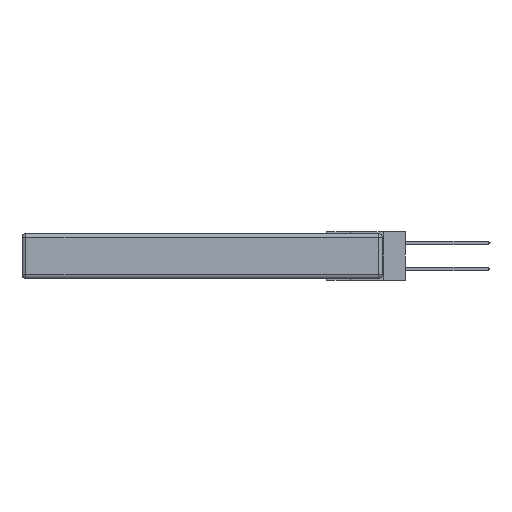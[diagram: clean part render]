
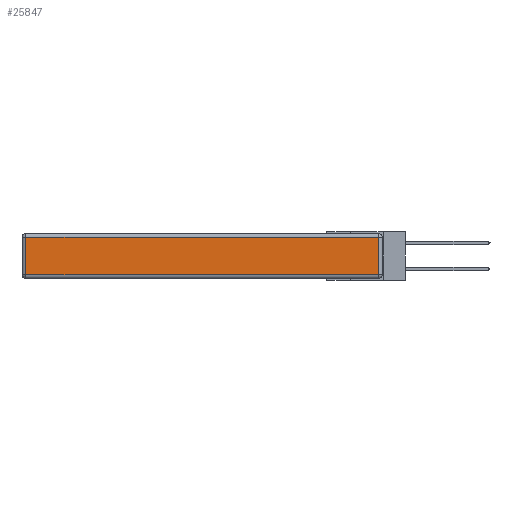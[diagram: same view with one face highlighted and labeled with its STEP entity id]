
A CAD part, left-side view. The second image highlights one B-rep face of the part: STEP entity #25847.
In plain terms, the highlighted planar face has unit normal (-1, 0, 0).
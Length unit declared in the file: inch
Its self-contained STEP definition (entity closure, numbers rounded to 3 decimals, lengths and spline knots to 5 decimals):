
#331 = DIRECTION ( 'NONE',  ( -1., 0., 0. ) ) ;
#1033 = CARTESIAN_POINT ( 'NONE',  ( 0., 0.03, -0.03 ) ) ;
#2004 = EDGE_CURVE ( 'NONE', #24551, #17968, #24460, .T. ) ;
#2163 = VERTEX_POINT ( 'NONE', #9667 ) ;
#3078 = FACE_OUTER_BOUND ( 'NONE', #28314, .T. ) ;
#4848 = VECTOR ( 'NONE', #13056, 39.37008 ) ;
#5954 = DIRECTION ( 'NONE',  ( 0., 0., 1. ) ) ;
#6379 = ORIENTED_EDGE ( 'NONE', *, *, #10879, .T. ) ;
#6501 = DIRECTION ( 'NONE',  ( 0., 1., 0. ) ) ;
#6529 = CARTESIAN_POINT ( 'NONE',  ( 0., 2.72, -0.313 ) ) ;
#8451 = ORIENTED_EDGE ( 'NONE', *, *, #25725, .T. ) ;
#9231 = CARTESIAN_POINT ( 'NONE',  ( 0., 0.03, -0.313 ) ) ;
#9667 = CARTESIAN_POINT ( 'NONE',  ( 0., 2.72, -0.03 ) ) ;
#9708 = CARTESIAN_POINT ( 'NONE',  ( 0., 2.72, -0.343 ) ) ;
#10006 = EDGE_CURVE ( 'NONE', #17968, #2163, #14911, .T. ) ;
#10088 = ORIENTED_EDGE ( 'NONE', *, *, #10006, .T. ) ;
#10879 = EDGE_CURVE ( 'NONE', #2163, #28955, #28136, .T. ) ;
#13056 = DIRECTION ( 'NONE',  ( 0., -1., 0. ) ) ;
#13531 = CARTESIAN_POINT ( 'NONE',  ( 0., 0., -0.343 ) ) ;
#14911 = LINE ( 'NONE', #17691, #15933 ) ;
#15243 = VECTOR ( 'NONE', #19004, 39.37008 ) ;
#15933 = VECTOR ( 'NONE', #6501, 39.37008 ) ;
#16073 = DIRECTION ( 'NONE',  ( 0., 0., 1. ) ) ;
#17159 = VECTOR ( 'NONE', #5954, 39.37008 ) ;
#17691 = CARTESIAN_POINT ( 'NONE',  ( 0., 2.75, -0.03 ) ) ;
#17968 = VERTEX_POINT ( 'NONE', #1033 ) ;
#18281 = PLANE ( 'NONE',  #22655 ) ;
#18297 = ORIENTED_EDGE ( 'NONE', *, *, #2004, .T. ) ;
#19004 = DIRECTION ( 'NONE',  ( 0., 0., -1. ) ) ;
#19976 = CARTESIAN_POINT ( 'NONE',  ( 0., 0., -0.313 ) ) ;
#21334 = LINE ( 'NONE', #19976, #4848 ) ;
#21914 = CARTESIAN_POINT ( 'NONE',  ( 0., 0.03, -0.343 ) ) ;
#22655 = AXIS2_PLACEMENT_3D ( 'NONE', #13531, #331, #16073 ) ;
#24460 = LINE ( 'NONE', #21914, #17159 ) ;
#24551 = VERTEX_POINT ( 'NONE', #9231 ) ;
#25725 = EDGE_CURVE ( 'NONE', #28955, #24551, #21334, .T. ) ;
#25847 = ADVANCED_FACE ( 'NONE', ( #3078 ), #18281, .T. ) ;
#28136 = LINE ( 'NONE', #9708, #15243 ) ;
#28314 = EDGE_LOOP ( 'NONE', ( #8451, #18297, #10088, #6379 ) ) ;
#28955 = VERTEX_POINT ( 'NONE', #6529 ) ;
